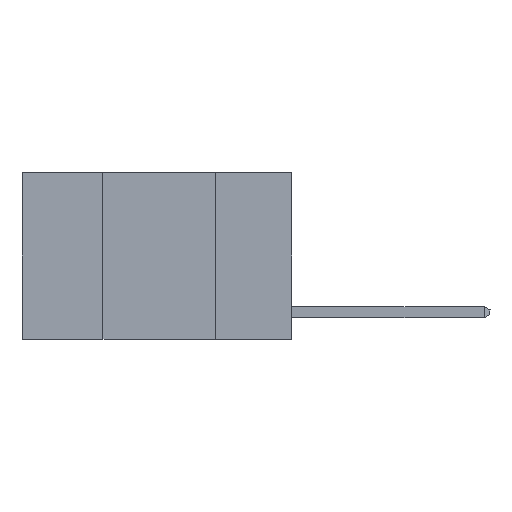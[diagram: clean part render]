
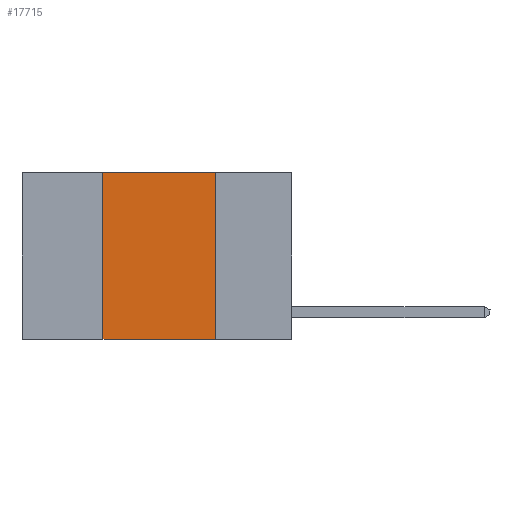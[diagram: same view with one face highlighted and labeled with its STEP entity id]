
A CAD part, left-side view. The second image highlights one B-rep face of the part: STEP entity #17715.
In plain terms, the highlighted planar face has unit normal (-1, 0, 0).
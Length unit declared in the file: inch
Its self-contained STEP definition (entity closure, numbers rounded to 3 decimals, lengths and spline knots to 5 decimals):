
#318 = VECTOR ( 'NONE', #9038, 39.37008 ) ;
#1090 = VERTEX_POINT ( 'NONE', #19068 ) ;
#1204 = LINE ( 'NONE', #8734, #14654 ) ;
#1581 = DIRECTION ( 'NONE',  ( 0., -1., 0. ) ) ;
#2673 = ORIENTED_EDGE ( 'NONE', *, *, #22908, .F. ) ;
#3066 = CARTESIAN_POINT ( 'NONE',  ( 0., 0.42, 0. ) ) ;
#3168 = LINE ( 'NONE', #17103, #19603 ) ;
#6056 = EDGE_CURVE ( 'NONE', #1090, #13101, #3168, .T. ) ;
#6361 = FACE_OUTER_BOUND ( 'NONE', #18305, .T. ) ;
#6491 = ORIENTED_EDGE ( 'NONE', *, *, #6056, .F. ) ;
#6996 = CARTESIAN_POINT ( 'NONE',  ( 0., 0.6, -0.37 ) ) ;
#8354 = DIRECTION ( 'NONE',  ( 0., 0., -1. ) ) ;
#8642 = CARTESIAN_POINT ( 'NONE',  ( 0., 0.42, -0.37 ) ) ;
#8734 = CARTESIAN_POINT ( 'NONE',  ( 0., 0.17, 0. ) ) ;
#8929 = VERTEX_POINT ( 'NONE', #18568 ) ;
#9038 = DIRECTION ( 'NONE',  ( 0., -1., 0. ) ) ;
#9305 = VERTEX_POINT ( 'NONE', #8642 ) ;
#9991 = ORIENTED_EDGE ( 'NONE', *, *, #20174, .T. ) ;
#11570 = LINE ( 'NONE', #3066, #18443 ) ;
#12757 = AXIS2_PLACEMENT_3D ( 'NONE', #17571, #13544, #8354 ) ;
#13101 = VERTEX_POINT ( 'NONE', #22406 ) ;
#13469 = EDGE_CURVE ( 'NONE', #13101, #8929, #1204, .T. ) ;
#13544 = DIRECTION ( 'NONE',  ( 1., 0., 0. ) ) ;
#14654 = VECTOR ( 'NONE', #22145, 39.37008 ) ;
#16350 = DIRECTION ( 'NONE',  ( 0., 0., 1. ) ) ;
#17103 = CARTESIAN_POINT ( 'NONE',  ( 0., 0.6, 0. ) ) ;
#17571 = CARTESIAN_POINT ( 'NONE',  ( 0., 0.6, 0. ) ) ;
#17715 = ADVANCED_FACE ( 'NONE', ( #6361 ), #23034, .F. ) ;
#18263 = LINE ( 'NONE', #6996, #318 ) ;
#18305 = EDGE_LOOP ( 'NONE', ( #22817, #6491, #2673, #9991 ) ) ;
#18443 = VECTOR ( 'NONE', #16350, 39.37008 ) ;
#18568 = CARTESIAN_POINT ( 'NONE',  ( 0., 0.17, -0.37 ) ) ;
#19068 = CARTESIAN_POINT ( 'NONE',  ( 0., 0.42, 0. ) ) ;
#19603 = VECTOR ( 'NONE', #1581, 39.37008 ) ;
#20174 = EDGE_CURVE ( 'NONE', #9305, #8929, #18263, .T. ) ;
#22145 = DIRECTION ( 'NONE',  ( 0., 0., -1. ) ) ;
#22406 = CARTESIAN_POINT ( 'NONE',  ( 0., 0.17, 0. ) ) ;
#22817 = ORIENTED_EDGE ( 'NONE', *, *, #13469, .F. ) ;
#22908 = EDGE_CURVE ( 'NONE', #9305, #1090, #11570, .T. ) ;
#23034 = PLANE ( 'NONE',  #12757 ) ;
